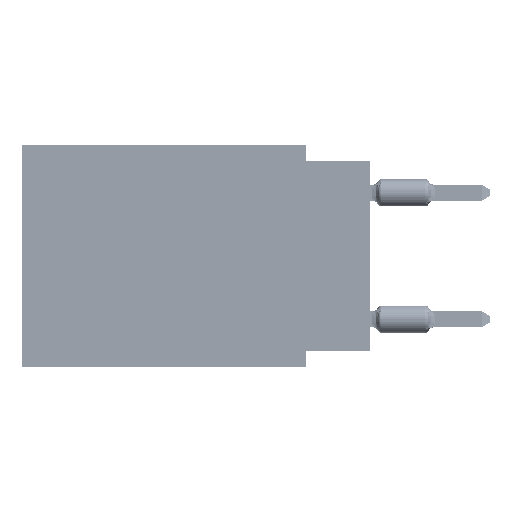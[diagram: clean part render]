
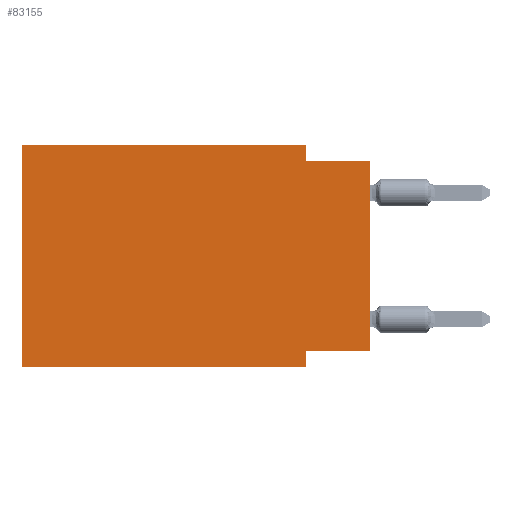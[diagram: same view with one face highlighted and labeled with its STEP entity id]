
A CAD part, left-side view. The second image highlights one B-rep face of the part: STEP entity #83155.
In plain terms, the highlighted planar face has unit normal (-1, 0, 0).
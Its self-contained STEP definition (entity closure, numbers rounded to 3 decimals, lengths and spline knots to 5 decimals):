
#5787 = EDGE_CURVE ( 'NONE', #52161, #15545, #34385, .T. ) ;
#7836 = DIRECTION ( 'NONE',  ( 0., 0., 1. ) ) ;
#8901 = PLANE ( 'NONE',  #17342 ) ;
#10118 = CARTESIAN_POINT ( 'NONE',  ( 0., 0.1, 0. ) ) ;
#11804 = ORIENTED_EDGE ( 'NONE', *, *, #49732, .F. ) ;
#15232 = LINE ( 'NONE', #63826, #73474 ) ;
#15444 = CARTESIAN_POINT ( 'NONE',  ( 0., 0., -0.325 ) ) ;
#15545 = VERTEX_POINT ( 'NONE', #76489 ) ;
#16914 = DIRECTION ( 'NONE',  ( 0., 0., -1. ) ) ;
#17342 = AXIS2_PLACEMENT_3D ( 'NONE', #101906, #19347, #16914 ) ;
#19347 = DIRECTION ( 'NONE',  ( 1., 0., 0. ) ) ;
#21747 = ORIENTED_EDGE ( 'NONE', *, *, #33510, .F. ) ;
#22619 = CARTESIAN_POINT ( 'NONE',  ( 0., 0., -0.025 ) ) ;
#27330 = VERTEX_POINT ( 'NONE', #60816 ) ;
#27487 = ORIENTED_EDGE ( 'NONE', *, *, #61529, .F. ) ;
#28004 = FACE_OUTER_BOUND ( 'NONE', #29738, .T. ) ;
#29738 = EDGE_LOOP ( 'NONE', ( #66697, #21747, #112174, #27487, #114417, #74900, #11804, #81202 ) ) ;
#33510 = EDGE_CURVE ( 'NONE', #15545, #91821, #89119, .T. ) ;
#34385 = LINE ( 'NONE', #108887, #49496 ) ;
#36045 = DIRECTION ( 'NONE',  ( 0., -1., 0. ) ) ;
#37402 = VERTEX_POINT ( 'NONE', #114121 ) ;
#38925 = VECTOR ( 'NONE', #42323, 39.37008 ) ;
#38983 = VERTEX_POINT ( 'NONE', #120825 ) ;
#42323 = DIRECTION ( 'NONE',  ( 0., -1., 0. ) ) ;
#43924 = CARTESIAN_POINT ( 'NONE',  ( 0., 0., 0. ) ) ;
#44541 = LINE ( 'NONE', #43924, #69291 ) ;
#45012 = DIRECTION ( 'NONE',  ( 0., 1., 0. ) ) ;
#49496 = VECTOR ( 'NONE', #81163, 39.37008 ) ;
#49732 = EDGE_CURVE ( 'NONE', #87586, #27330, #68958, .T. ) ;
#52161 = VERTEX_POINT ( 'NONE', #10118 ) ;
#53605 = LINE ( 'NONE', #15444, #79223 ) ;
#54501 = LINE ( 'NONE', #83418, #99768 ) ;
#57652 = CARTESIAN_POINT ( 'NONE',  ( 0., 0., -0.025 ) ) ;
#60816 = CARTESIAN_POINT ( 'NONE',  ( 0., 0.1, -0.35 ) ) ;
#61529 = EDGE_CURVE ( 'NONE', #80803, #52161, #92086, .T. ) ;
#63826 = CARTESIAN_POINT ( 'NONE',  ( 0., 0.55, 0. ) ) ;
#66697 = ORIENTED_EDGE ( 'NONE', *, *, #102156, .T. ) ;
#66951 = EDGE_CURVE ( 'NONE', #37402, #27330, #54501, .T. ) ;
#68958 = LINE ( 'NONE', #115159, #88296 ) ;
#69291 = VECTOR ( 'NONE', #81450, 39.37008 ) ;
#73474 = VECTOR ( 'NONE', #7836, 39.37008 ) ;
#74900 = ORIENTED_EDGE ( 'NONE', *, *, #66951, .T. ) ;
#75831 = DIRECTION ( 'NONE',  ( 0., -1., 0. ) ) ;
#76489 = CARTESIAN_POINT ( 'NONE',  ( 0., 0.1, -0.025 ) ) ;
#78739 = CARTESIAN_POINT ( 'NONE',  ( 0., 0.1, -0.325 ) ) ;
#79223 = VECTOR ( 'NONE', #45012, 39.37008 ) ;
#79409 = CARTESIAN_POINT ( 'NONE',  ( 0., 0.55, 0. ) ) ;
#80803 = VERTEX_POINT ( 'NONE', #79409 ) ;
#81163 = DIRECTION ( 'NONE',  ( 0., 0., -1. ) ) ;
#81202 = ORIENTED_EDGE ( 'NONE', *, *, #102698, .F. ) ;
#81450 = DIRECTION ( 'NONE',  ( 0., 0., 1. ) ) ;
#83155 = ADVANCED_FACE ( 'NONE', ( #28004 ), #8901, .F. ) ;
#83418 = CARTESIAN_POINT ( 'NONE',  ( 0., 0.55, -0.35 ) ) ;
#87586 = VERTEX_POINT ( 'NONE', #78739 ) ;
#88296 = VECTOR ( 'NONE', #107140, 39.37008 ) ;
#89119 = LINE ( 'NONE', #22619, #38925 ) ;
#91821 = VERTEX_POINT ( 'NONE', #57652 ) ;
#92086 = LINE ( 'NONE', #111139, #116917 ) ;
#99768 = VECTOR ( 'NONE', #75831, 39.37008 ) ;
#101906 = CARTESIAN_POINT ( 'NONE',  ( 0., 0.55, 0. ) ) ;
#102156 = EDGE_CURVE ( 'NONE', #38983, #91821, #44541, .T. ) ;
#102698 = EDGE_CURVE ( 'NONE', #38983, #87586, #53605, .T. ) ;
#107140 = DIRECTION ( 'NONE',  ( 0., 0., -1. ) ) ;
#108887 = CARTESIAN_POINT ( 'NONE',  ( 0., 0.1, 0. ) ) ;
#110934 = EDGE_CURVE ( 'NONE', #37402, #80803, #15232, .T. ) ;
#111139 = CARTESIAN_POINT ( 'NONE',  ( 0., 0.55, 0. ) ) ;
#112174 = ORIENTED_EDGE ( 'NONE', *, *, #5787, .F. ) ;
#114121 = CARTESIAN_POINT ( 'NONE',  ( 0., 0.55, -0.35 ) ) ;
#114417 = ORIENTED_EDGE ( 'NONE', *, *, #110934, .F. ) ;
#115159 = CARTESIAN_POINT ( 'NONE',  ( 0., 0.1, -0.35 ) ) ;
#116917 = VECTOR ( 'NONE', #36045, 39.37008 ) ;
#120825 = CARTESIAN_POINT ( 'NONE',  ( 0., 0., -0.325 ) ) ;
